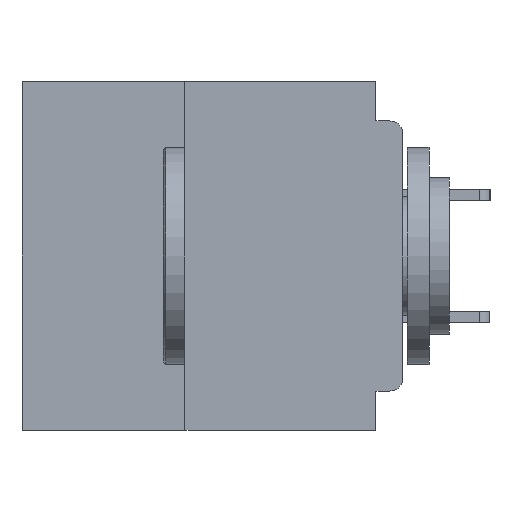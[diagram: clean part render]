
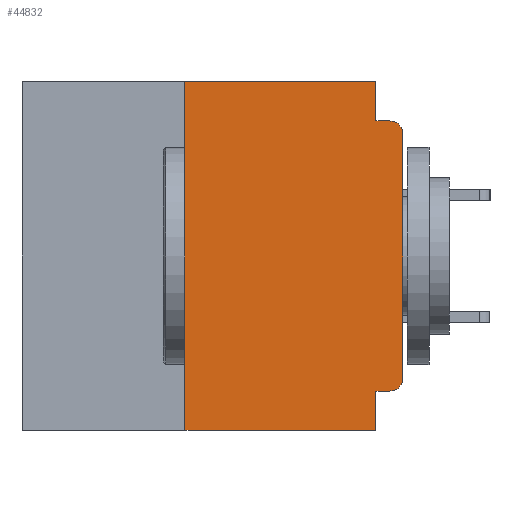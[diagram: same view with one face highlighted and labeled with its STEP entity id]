
A CAD part, left-side view. The second image highlights one B-rep face of the part: STEP entity #44832.
In plain terms, the highlighted planar face has unit normal (-1, 0, 0).
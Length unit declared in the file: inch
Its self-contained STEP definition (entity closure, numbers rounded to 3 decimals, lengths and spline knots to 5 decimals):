
#3961 = CARTESIAN_POINT ( 'NONE',  ( 0., 0.031, -0.4 ) ) ;
#4134 = DIRECTION ( 'NONE',  ( 0., 0., -1. ) ) ;
#4609 = CARTESIAN_POINT ( 'NONE',  ( 0., 0.031, -0.4 ) ) ;
#5541 = CIRCLE ( 'NONE', #21435, 0.015 ) ;
#6014 = LINE ( 'NONE', #41910, #39702 ) ;
#6406 = LINE ( 'NONE', #48852, #29390 ) ;
#6534 = CARTESIAN_POINT ( 'NONE',  ( 0., 0.25, -0.4 ) ) ;
#6867 = VECTOR ( 'NONE', #28124, 39.37008 ) ;
#7810 = VERTEX_POINT ( 'NONE', #15187 ) ;
#8083 = PLANE ( 'NONE',  #26295 ) ;
#9106 = DIRECTION ( 'NONE',  ( 0., -1., 0. ) ) ;
#9182 = EDGE_LOOP ( 'NONE', ( #49552, #53386, #24120, #32224, #15642, #32278, #50093, #32636, #43393, #56238 ) ) ;
#11408 = VERTEX_POINT ( 'NONE', #39202 ) ;
#12060 = VECTOR ( 'NONE', #36063, 39.37008 ) ;
#12705 = DIRECTION ( 'NONE',  ( 1., 0., 0. ) ) ;
#15187 = CARTESIAN_POINT ( 'NONE',  ( 0., 0.015, -0.045 ) ) ;
#15642 = ORIENTED_EDGE ( 'NONE', *, *, #49793, .F. ) ;
#16679 = DIRECTION ( 'NONE',  ( -1., 0., 0. ) ) ;
#18245 = VERTEX_POINT ( 'NONE', #45156 ) ;
#19141 = LINE ( 'NONE', #46295, #6867 ) ;
#20644 = VERTEX_POINT ( 'NONE', #50396 ) ;
#20681 = CARTESIAN_POINT ( 'NONE',  ( 0., 0.25, -0.4 ) ) ;
#21435 = AXIS2_PLACEMENT_3D ( 'NONE', #44063, #16679, #48677 ) ;
#22887 = LINE ( 'NONE', #3961, #12060 ) ;
#24120 = ORIENTED_EDGE ( 'NONE', *, *, #34175, .F. ) ;
#24522 = EDGE_CURVE ( 'NONE', #18245, #44987, #22887, .T. ) ;
#24557 = CARTESIAN_POINT ( 'NONE',  ( 0., 0.015, -0.355 ) ) ;
#25261 = DIRECTION ( 'NONE',  ( 0., 0., 1. ) ) ;
#26083 = DIRECTION ( 'NONE',  ( 0., 1., 0. ) ) ;
#26146 = DIRECTION ( 'NONE',  ( 0., 0., 1. ) ) ;
#26271 = CARTESIAN_POINT ( 'NONE',  ( 0., 0., -0.06 ) ) ;
#26295 = AXIS2_PLACEMENT_3D ( 'NONE', #53723, #12705, #44739 ) ;
#27250 = VECTOR ( 'NONE', #25261, 39.37008 ) ;
#28124 = DIRECTION ( 'NONE',  ( 0., 0., -1. ) ) ;
#28675 = LINE ( 'NONE', #20681, #27250 ) ;
#29143 = VERTEX_POINT ( 'NONE', #26271 ) ;
#29243 = EDGE_CURVE ( 'NONE', #49452, #20644, #28675, .T. ) ;
#29390 = VECTOR ( 'NONE', #26083, 39.37008 ) ;
#30409 = VERTEX_POINT ( 'NONE', #24557 ) ;
#31094 = FACE_OUTER_BOUND ( 'NONE', #9182, .T. ) ;
#31668 = DIRECTION ( 'NONE',  ( -1., 0., 0. ) ) ;
#32224 = ORIENTED_EDGE ( 'NONE', *, *, #48567, .F. ) ;
#32278 = ORIENTED_EDGE ( 'NONE', *, *, #29243, .F. ) ;
#32636 = ORIENTED_EDGE ( 'NONE', *, *, #24522, .F. ) ;
#32785 = LINE ( 'NONE', #44523, #34199 ) ;
#34175 = EDGE_CURVE ( 'NONE', #53954, #7810, #37843, .T. ) ;
#34199 = VECTOR ( 'NONE', #26146, 39.37008 ) ;
#35261 = EDGE_CURVE ( 'NONE', #30409, #56103, #5541, .T. ) ;
#36063 = DIRECTION ( 'NONE',  ( 0., 0., -1. ) ) ;
#36426 = VECTOR ( 'NONE', #45806, 39.37008 ) ;
#37086 = DIRECTION ( 'NONE',  ( 0., -1., 0. ) ) ;
#37630 = VECTOR ( 'NONE', #9106, 39.37008 ) ;
#37843 = LINE ( 'NONE', #54586, #36426 ) ;
#38566 = CARTESIAN_POINT ( 'NONE',  ( 0., 0.031, -0.045 ) ) ;
#39202 = CARTESIAN_POINT ( 'NONE',  ( 0., 0.031, 0. ) ) ;
#39702 = VECTOR ( 'NONE', #37086, 39.37008 ) ;
#40967 = CARTESIAN_POINT ( 'NONE',  ( 0., 0.437, 0. ) ) ;
#40984 = AXIS2_PLACEMENT_3D ( 'NONE', #59004, #31668, #4134 ) ;
#41910 = CARTESIAN_POINT ( 'NONE',  ( 0., 0.437, -0.4 ) ) ;
#43393 = ORIENTED_EDGE ( 'NONE', *, *, #56074, .F. ) ;
#44063 = CARTESIAN_POINT ( 'NONE',  ( 0., 0.015, -0.34 ) ) ;
#44523 = CARTESIAN_POINT ( 'NONE',  ( 0., 0., 0. ) ) ;
#44739 = DIRECTION ( 'NONE',  ( 0., 0., -1. ) ) ;
#44832 = ADVANCED_FACE ( 'NONE', ( #31094 ), #8083, .F. ) ;
#44987 = VERTEX_POINT ( 'NONE', #4609 ) ;
#45156 = CARTESIAN_POINT ( 'NONE',  ( 0., 0.031, -0.355 ) ) ;
#45806 = DIRECTION ( 'NONE',  ( 0., -1., 0. ) ) ;
#46295 = CARTESIAN_POINT ( 'NONE',  ( 0., 0.031, 0. ) ) ;
#48097 = EDGE_CURVE ( 'NONE', #56103, #29143, #32785, .T. ) ;
#48567 = EDGE_CURVE ( 'NONE', #11408, #53954, #19141, .T. ) ;
#48677 = DIRECTION ( 'NONE',  ( 0., 0., -1. ) ) ;
#48852 = CARTESIAN_POINT ( 'NONE',  ( 0., 0., -0.355 ) ) ;
#49075 = EDGE_CURVE ( 'NONE', #29143, #7810, #53477, .T. ) ;
#49452 = VERTEX_POINT ( 'NONE', #6534 ) ;
#49552 = ORIENTED_EDGE ( 'NONE', *, *, #48097, .T. ) ;
#49793 = EDGE_CURVE ( 'NONE', #20644, #11408, #49822, .T. ) ;
#49822 = LINE ( 'NONE', #40967, #37630 ) ;
#50093 = ORIENTED_EDGE ( 'NONE', *, *, #50437, .T. ) ;
#50396 = CARTESIAN_POINT ( 'NONE',  ( 0., 0.25, 0. ) ) ;
#50437 = EDGE_CURVE ( 'NONE', #49452, #44987, #6014, .T. ) ;
#52014 = CARTESIAN_POINT ( 'NONE',  ( 0., 0., -0.34 ) ) ;
#53386 = ORIENTED_EDGE ( 'NONE', *, *, #49075, .T. ) ;
#53477 = CIRCLE ( 'NONE', #40984, 0.015 ) ;
#53723 = CARTESIAN_POINT ( 'NONE',  ( 0., 0.437, 0. ) ) ;
#53954 = VERTEX_POINT ( 'NONE', #38566 ) ;
#54586 = CARTESIAN_POINT ( 'NONE',  ( 0., 0., -0.045 ) ) ;
#56074 = EDGE_CURVE ( 'NONE', #30409, #18245, #6406, .T. ) ;
#56103 = VERTEX_POINT ( 'NONE', #52014 ) ;
#56238 = ORIENTED_EDGE ( 'NONE', *, *, #35261, .T. ) ;
#59004 = CARTESIAN_POINT ( 'NONE',  ( 0., 0.015, -0.06 ) ) ;
